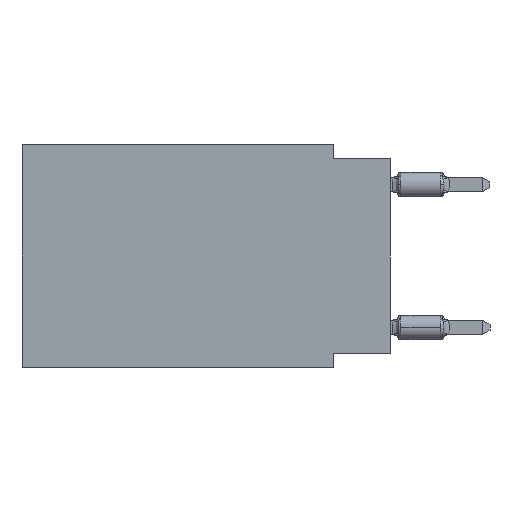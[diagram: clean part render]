
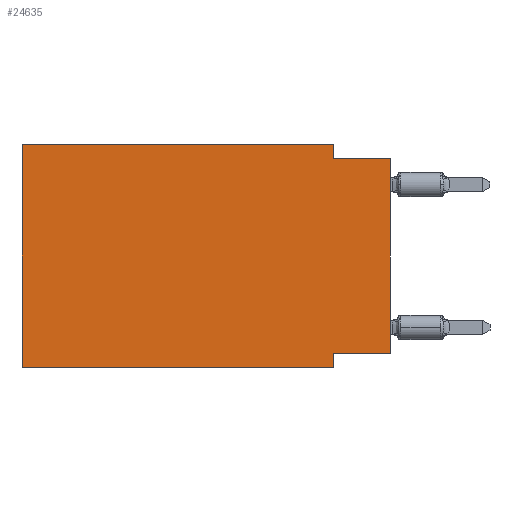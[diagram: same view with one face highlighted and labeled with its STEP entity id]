
A CAD part, left-side view. The second image highlights one B-rep face of the part: STEP entity #24635.
In plain terms, the highlighted planar face has unit normal (-1, 0, 0).
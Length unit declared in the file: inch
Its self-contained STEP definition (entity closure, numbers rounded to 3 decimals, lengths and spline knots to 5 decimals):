
#305 = CARTESIAN_POINT ( 'NONE',  ( 0., 0.645, -0.39 ) ) ;
#734 = ORIENTED_EDGE ( 'NONE', *, *, #38201, .F. ) ;
#1008 = DIRECTION ( 'NONE',  ( 0., 1., 0. ) ) ;
#1172 = VECTOR ( 'NONE', #20930, 39.37008 ) ;
#2876 = LINE ( 'NONE', #5224, #17057 ) ;
#2885 = LINE ( 'NONE', #23863, #15825 ) ;
#2980 = CARTESIAN_POINT ( 'NONE',  ( 0., 0.645, 0. ) ) ;
#3519 = CARTESIAN_POINT ( 'NONE',  ( 0., 0., -0.365 ) ) ;
#3817 = LINE ( 'NONE', #24994, #15555 ) ;
#4939 = CARTESIAN_POINT ( 'NONE',  ( 0., 0.1, -0.39 ) ) ;
#5022 = PLANE ( 'NONE',  #24746 ) ;
#5119 = LINE ( 'NONE', #4939, #21796 ) ;
#5224 = CARTESIAN_POINT ( 'NONE',  ( 0., 0.1, 0. ) ) ;
#5405 = CARTESIAN_POINT ( 'NONE',  ( 0., 0.1, -0.025 ) ) ;
#5726 = CARTESIAN_POINT ( 'NONE',  ( 0., 0.1, 0. ) ) ;
#5750 = VERTEX_POINT ( 'NONE', #19496 ) ;
#6326 = EDGE_CURVE ( 'NONE', #33566, #9135, #11652, .T. ) ;
#6489 = EDGE_CURVE ( 'NONE', #34961, #9135, #3817, .T. ) ;
#6603 = ORIENTED_EDGE ( 'NONE', *, *, #37350, .F. ) ;
#6988 = CARTESIAN_POINT ( 'NONE',  ( 0., 0.1, -0.365 ) ) ;
#7684 = VECTOR ( 'NONE', #8630, 39.37008 ) ;
#7756 = DIRECTION ( 'NONE',  ( 1., 0., 0. ) ) ;
#8247 = LINE ( 'NONE', #2980, #7684 ) ;
#8630 = DIRECTION ( 'NONE',  ( 0., -1., 0. ) ) ;
#9135 = VERTEX_POINT ( 'NONE', #35090 ) ;
#9296 = DIRECTION ( 'NONE',  ( 0., 0., 1. ) ) ;
#10695 = VERTEX_POINT ( 'NONE', #5726 ) ;
#11560 = EDGE_LOOP ( 'NONE', ( #17756, #18707, #24760, #22369, #6603, #27496, #15966, #734 ) ) ;
#11652 = LINE ( 'NONE', #16898, #30430 ) ;
#11828 = DIRECTION ( 'NONE',  ( 0., 0., -1. ) ) ;
#14318 = EDGE_CURVE ( 'NONE', #10695, #33566, #2876, .T. ) ;
#15183 = LINE ( 'NONE', #3519, #23850 ) ;
#15555 = VECTOR ( 'NONE', #17065, 39.37008 ) ;
#15825 = VECTOR ( 'NONE', #9296, 39.37008 ) ;
#15966 = ORIENTED_EDGE ( 'NONE', *, *, #29651, .F. ) ;
#16874 = DIRECTION ( 'NONE',  ( 0., 0., -1. ) ) ;
#16898 = CARTESIAN_POINT ( 'NONE',  ( 0., 0., -0.025 ) ) ;
#17057 = VECTOR ( 'NONE', #11828, 39.37008 ) ;
#17065 = DIRECTION ( 'NONE',  ( 0., 0., 1. ) ) ;
#17756 = ORIENTED_EDGE ( 'NONE', *, *, #6489, .T. ) ;
#18707 = ORIENTED_EDGE ( 'NONE', *, *, #6326, .F. ) ;
#19203 = CARTESIAN_POINT ( 'NONE',  ( 0., 0.645, 0. ) ) ;
#19231 = FACE_OUTER_BOUND ( 'NONE', #11560, .T. ) ;
#19496 = CARTESIAN_POINT ( 'NONE',  ( 0., 0.1, -0.39 ) ) ;
#20930 = DIRECTION ( 'NONE',  ( 0., -1., 0. ) ) ;
#21383 = VERTEX_POINT ( 'NONE', #6988 ) ;
#21796 = VECTOR ( 'NONE', #29177, 39.37008 ) ;
#22369 = ORIENTED_EDGE ( 'NONE', *, *, #36325, .F. ) ;
#23293 = DIRECTION ( 'NONE',  ( 0., -1., 0. ) ) ;
#23850 = VECTOR ( 'NONE', #1008, 39.37008 ) ;
#23863 = CARTESIAN_POINT ( 'NONE',  ( 0., 0.645, 0. ) ) ;
#24635 = ADVANCED_FACE ( 'NONE', ( #19231 ), #5022, .F. ) ;
#24711 = EDGE_CURVE ( 'NONE', #27662, #5750, #32388, .T. ) ;
#24746 = AXIS2_PLACEMENT_3D ( 'NONE', #31816, #7756, #16874 ) ;
#24760 = ORIENTED_EDGE ( 'NONE', *, *, #14318, .F. ) ;
#24994 = CARTESIAN_POINT ( 'NONE',  ( 0., 0., 0. ) ) ;
#27496 = ORIENTED_EDGE ( 'NONE', *, *, #24711, .T. ) ;
#27662 = VERTEX_POINT ( 'NONE', #305 ) ;
#29177 = DIRECTION ( 'NONE',  ( 0., 0., -1. ) ) ;
#29651 = EDGE_CURVE ( 'NONE', #21383, #5750, #5119, .T. ) ;
#30430 = VECTOR ( 'NONE', #23293, 39.37008 ) ;
#31816 = CARTESIAN_POINT ( 'NONE',  ( 0., 0.645, 0. ) ) ;
#32388 = LINE ( 'NONE', #38016, #1172 ) ;
#32774 = CARTESIAN_POINT ( 'NONE',  ( 0., 0., -0.365 ) ) ;
#33566 = VERTEX_POINT ( 'NONE', #5405 ) ;
#34961 = VERTEX_POINT ( 'NONE', #32774 ) ;
#35086 = VERTEX_POINT ( 'NONE', #19203 ) ;
#35090 = CARTESIAN_POINT ( 'NONE',  ( 0., 0., -0.025 ) ) ;
#36325 = EDGE_CURVE ( 'NONE', #35086, #10695, #8247, .T. ) ;
#37350 = EDGE_CURVE ( 'NONE', #27662, #35086, #2885, .T. ) ;
#38016 = CARTESIAN_POINT ( 'NONE',  ( 0., 0.645, -0.39 ) ) ;
#38201 = EDGE_CURVE ( 'NONE', #34961, #21383, #15183, .T. ) ;
